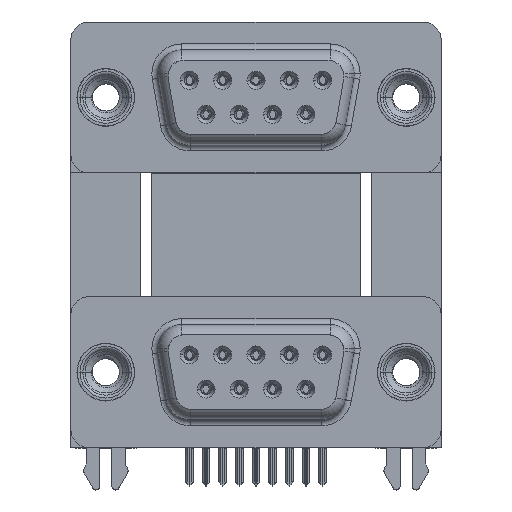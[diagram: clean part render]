
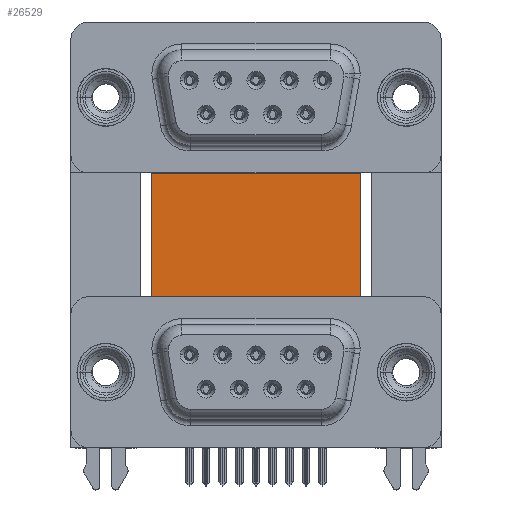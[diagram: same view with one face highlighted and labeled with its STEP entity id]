
A CAD part, top view. The second image highlights one B-rep face of the part: STEP entity #26529.
In plain terms, the highlighted planar face has unit normal (0, 0, 1).
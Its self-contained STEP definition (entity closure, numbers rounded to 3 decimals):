
#1694 = CARTESIAN_POINT ( 'NONE',  ( 22.59, -4.635, -12. ) ) ;
#2067 = VECTOR ( 'NONE', #43791, 1000. ) ;
#2139 = VERTEX_POINT ( 'NONE', #18238 ) ;
#2451 = CARTESIAN_POINT ( 'NONE',  ( 2.4, -4.635, -12. ) ) ;
#2573 = FACE_OUTER_BOUND ( 'NONE', #30085, .T. ) ;
#3452 = VERTEX_POINT ( 'NONE', #42557 ) ;
#3461 = LINE ( 'NONE', #10026, #16084 ) ;
#5329 = ORIENTED_EDGE ( 'NONE', *, *, #34273, .T. ) ;
#5507 = DIRECTION ( 'NONE',  ( -0.336, 0.942, 0. ) ) ;
#5867 = VERTEX_POINT ( 'NONE', #18948 ) ;
#6432 = ORIENTED_EDGE ( 'NONE', *, *, #22372, .F. ) ;
#6583 = VECTOR ( 'NONE', #26068, 1000. ) ;
#8400 = DIRECTION ( 'NONE',  ( 0., 1., 0. ) ) ;
#9600 = DIRECTION ( 'NONE',  ( 0., 0., -1. ) ) ;
#10026 = CARTESIAN_POINT ( 'NONE',  ( 21.2, 16.585, -12. ) ) ;
#10698 = VECTOR ( 'NONE', #14888, 1000. ) ;
#11072 = EDGE_CURVE ( 'NONE', #28877, #2139, #20472, .T. ) ;
#11461 = VERTEX_POINT ( 'NONE', #16799 ) ;
#12277 = CARTESIAN_POINT ( 'NONE',  ( 22.09, -3.735, -12. ) ) ;
#12280 = LINE ( 'NONE', #18844, #27544 ) ;
#12631 = CARTESIAN_POINT ( 'NONE',  ( 3.79, -3.735, -12. ) ) ;
#12964 = CARTESIAN_POINT ( 'NONE',  ( 3.79, 16.585, -12. ) ) ;
#13551 = ORIENTED_EDGE ( 'NONE', *, *, #35556, .F. ) ;
#14741 = VECTOR ( 'NONE', #44186, 1000. ) ;
#14888 = DIRECTION ( 'NONE',  ( 1., 0., 0. ) ) ;
#15437 = LINE ( 'NONE', #36444, #40446 ) ;
#16084 = VECTOR ( 'NONE', #37774, 1000. ) ;
#16107 = ORIENTED_EDGE ( 'NONE', *, *, #11072, .T. ) ;
#16277 = VERTEX_POINT ( 'NONE', #43175 ) ;
#16355 = PLANE ( 'NONE',  #36497 ) ;
#16799 = CARTESIAN_POINT ( 'NONE',  ( 2.4, -4.635, -12. ) ) ;
#18238 = CARTESIAN_POINT ( 'NONE',  ( 3.79, -0.735, -12. ) ) ;
#18398 = LINE ( 'NONE', #12277, #6583 ) ;
#18844 = CARTESIAN_POINT ( 'NONE',  ( 2.9, -4.635, -12. ) ) ;
#18920 = VERTEX_POINT ( 'NONE', #1694 ) ;
#18948 = CARTESIAN_POINT ( 'NONE',  ( 22.09, -4.635, -12. ) ) ;
#19632 = LINE ( 'NONE', #2451, #30901 ) ;
#20472 = LINE ( 'NONE', #30186, #14741 ) ;
#20883 = VECTOR ( 'NONE', #8400, 1000. ) ;
#22218 = CARTESIAN_POINT ( 'NONE',  ( 22.09, -4.635, -12. ) ) ;
#22372 = EDGE_CURVE ( 'NONE', #41723, #3452, #3461, .T. ) ;
#23307 = EDGE_CURVE ( 'NONE', #5867, #18920, #25634, .T. ) ;
#23346 = DIRECTION ( 'NONE',  ( -1., 0., 0. ) ) ;
#23695 = ORIENTED_EDGE ( 'NONE', *, *, #32730, .T. ) ;
#25634 = LINE ( 'NONE', #22218, #37809 ) ;
#26068 = DIRECTION ( 'NONE',  ( 0., -1., 0. ) ) ;
#26070 = DIRECTION ( 'NONE',  ( 1., 0., 0. ) ) ;
#26529 = ADVANCED_FACE ( 'NONE', ( #2573 ), #16355, .F. ) ;
#27544 = VECTOR ( 'NONE', #26070, 1000. ) ;
#28721 = LINE ( 'NONE', #32775, #20883 ) ;
#28877 = VERTEX_POINT ( 'NONE', #35052 ) ;
#29125 = CARTESIAN_POINT ( 'NONE',  ( 22.09, -3.735, -12. ) ) ;
#29311 = ORIENTED_EDGE ( 'NONE', *, *, #23307, .T. ) ;
#30085 = EDGE_LOOP ( 'NONE', ( #5329, #35009, #29311, #34160, #6432, #13551, #16107, #43347, #23695, #44022 ) ) ;
#30186 = CARTESIAN_POINT ( 'NONE',  ( 3.79, 16.585, -12. ) ) ;
#30901 = VECTOR ( 'NONE', #43782, 1000. ) ;
#31257 = EDGE_CURVE ( 'NONE', #18920, #3452, #15437, .T. ) ;
#31347 = EDGE_CURVE ( 'NONE', #33453, #5867, #18398, .T. ) ;
#31618 = CARTESIAN_POINT ( 'NONE',  ( 2.9, -3.735, -12. ) ) ;
#32730 = EDGE_CURVE ( 'NONE', #11461, #16277, #12280, .T. ) ;
#32775 = CARTESIAN_POINT ( 'NONE',  ( 2.9, -3.735, -12. ) ) ;
#33324 = VERTEX_POINT ( 'NONE', #31618 ) ;
#33453 = VERTEX_POINT ( 'NONE', #29125 ) ;
#34160 = ORIENTED_EDGE ( 'NONE', *, *, #31257, .T. ) ;
#34273 = EDGE_CURVE ( 'NONE', #33324, #33453, #40178, .T. ) ;
#34791 = CARTESIAN_POINT ( 'NONE',  ( 3.79, 16.585, -12. ) ) ;
#35009 = ORIENTED_EDGE ( 'NONE', *, *, #31347, .T. ) ;
#35052 = CARTESIAN_POINT ( 'NONE',  ( 3.79, 16.585, -12. ) ) ;
#35556 = EDGE_CURVE ( 'NONE', #28877, #41723, #41782, .T. ) ;
#35839 = EDGE_CURVE ( 'NONE', #2139, #11461, #19632, .T. ) ;
#36444 = CARTESIAN_POINT ( 'NONE',  ( 22.59, -4.635, -12. ) ) ;
#36497 = AXIS2_PLACEMENT_3D ( 'NONE', #12964, #9600, #23346 ) ;
#37774 = DIRECTION ( 'NONE',  ( 0., -1., 0. ) ) ;
#37809 = VECTOR ( 'NONE', #42340, 1000. ) ;
#40178 = LINE ( 'NONE', #12631, #2067 ) ;
#40446 = VECTOR ( 'NONE', #5507, 1000. ) ;
#41723 = VERTEX_POINT ( 'NONE', #43538 ) ;
#41782 = LINE ( 'NONE', #34791, #10698 ) ;
#42340 = DIRECTION ( 'NONE',  ( 1., 0., 0. ) ) ;
#42557 = CARTESIAN_POINT ( 'NONE',  ( 21.2, -0.735, -12. ) ) ;
#43175 = CARTESIAN_POINT ( 'NONE',  ( 2.9, -4.635, -12. ) ) ;
#43347 = ORIENTED_EDGE ( 'NONE', *, *, #35839, .T. ) ;
#43538 = CARTESIAN_POINT ( 'NONE',  ( 21.2, 16.585, -12. ) ) ;
#43782 = DIRECTION ( 'NONE',  ( -0.336, -0.942, 0. ) ) ;
#43791 = DIRECTION ( 'NONE',  ( 1., 0., 0. ) ) ;
#44022 = ORIENTED_EDGE ( 'NONE', *, *, #44107, .T. ) ;
#44107 = EDGE_CURVE ( 'NONE', #16277, #33324, #28721, .T. ) ;
#44186 = DIRECTION ( 'NONE',  ( 0., -1., 0. ) ) ;
